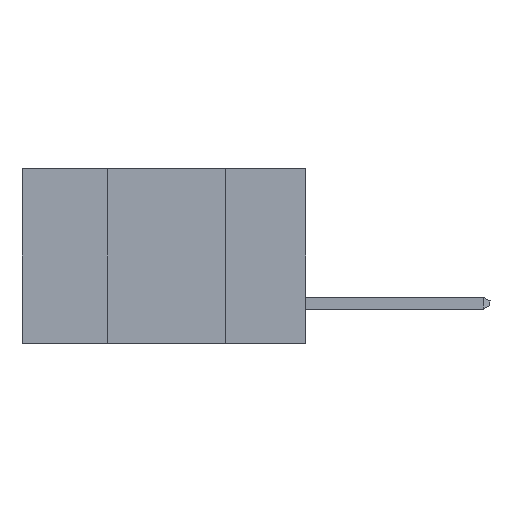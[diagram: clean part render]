
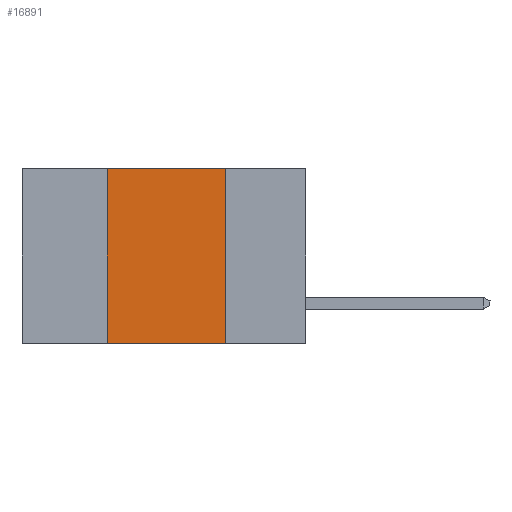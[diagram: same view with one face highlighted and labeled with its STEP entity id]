
A CAD part, left-side view. The second image highlights one B-rep face of the part: STEP entity #16891.
In plain terms, the highlighted planar face has unit normal (-1, 0, 0).
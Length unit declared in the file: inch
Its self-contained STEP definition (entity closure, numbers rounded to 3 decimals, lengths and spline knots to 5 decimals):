
#72 = VERTEX_POINT ( 'NONE', #10953 ) ;
#318 = VERTEX_POINT ( 'NONE', #17159 ) ;
#919 = CARTESIAN_POINT ( 'NONE',  ( 0., 0.6, 0. ) ) ;
#2684 = LINE ( 'NONE', #12585, #15339 ) ;
#2750 = FACE_OUTER_BOUND ( 'NONE', #18974, .T. ) ;
#2898 = AXIS2_PLACEMENT_3D ( 'NONE', #919, #17383, #19093 ) ;
#2921 = CARTESIAN_POINT ( 'NONE',  ( 0., 0.42, -0.37 ) ) ;
#3367 = EDGE_CURVE ( 'NONE', #318, #72, #2684, .T. ) ;
#3874 = VECTOR ( 'NONE', #17663, 39.37008 ) ;
#7144 = CARTESIAN_POINT ( 'NONE',  ( 0., 0.17, -0.37 ) ) ;
#7335 = VERTEX_POINT ( 'NONE', #21167 ) ;
#7853 = LINE ( 'NONE', #19232, #13702 ) ;
#8554 = ORIENTED_EDGE ( 'NONE', *, *, #12621, .F. ) ;
#9916 = EDGE_CURVE ( 'NONE', #72, #12378, #7853, .T. ) ;
#10204 = ORIENTED_EDGE ( 'NONE', *, *, #3367, .F. ) ;
#10284 = DIRECTION ( 'NONE',  ( 0., -1., 0. ) ) ;
#10880 = DIRECTION ( 'NONE',  ( 0., 0., -1. ) ) ;
#10953 = CARTESIAN_POINT ( 'NONE',  ( 0., 0.17, 0. ) ) ;
#11545 = LINE ( 'NONE', #2921, #3874 ) ;
#11781 = LINE ( 'NONE', #11892, #13128 ) ;
#11892 = CARTESIAN_POINT ( 'NONE',  ( 0., 0.6, -0.37 ) ) ;
#12378 = VERTEX_POINT ( 'NONE', #7144 ) ;
#12408 = EDGE_CURVE ( 'NONE', #7335, #12378, #11781, .T. ) ;
#12585 = CARTESIAN_POINT ( 'NONE',  ( 0., 0.6, 0. ) ) ;
#12621 = EDGE_CURVE ( 'NONE', #7335, #318, #11545, .T. ) ;
#13128 = VECTOR ( 'NONE', #10284, 39.37008 ) ;
#13702 = VECTOR ( 'NONE', #10880, 39.37008 ) ;
#15339 = VECTOR ( 'NONE', #19427, 39.37008 ) ;
#16891 = ADVANCED_FACE ( 'NONE', ( #2750 ), #19192, .F. ) ;
#17159 = CARTESIAN_POINT ( 'NONE',  ( 0., 0.42, 0. ) ) ;
#17383 = DIRECTION ( 'NONE',  ( 1., 0., 0. ) ) ;
#17663 = DIRECTION ( 'NONE',  ( 0., 0., 1. ) ) ;
#18974 = EDGE_LOOP ( 'NONE', ( #19671, #10204, #8554, #20255 ) ) ;
#19093 = DIRECTION ( 'NONE',  ( 0., 0., -1. ) ) ;
#19192 = PLANE ( 'NONE',  #2898 ) ;
#19232 = CARTESIAN_POINT ( 'NONE',  ( 0., 0.17, -0.37 ) ) ;
#19427 = DIRECTION ( 'NONE',  ( 0., -1., 0. ) ) ;
#19671 = ORIENTED_EDGE ( 'NONE', *, *, #9916, .F. ) ;
#20255 = ORIENTED_EDGE ( 'NONE', *, *, #12408, .T. ) ;
#21167 = CARTESIAN_POINT ( 'NONE',  ( 0., 0.42, -0.37 ) ) ;
